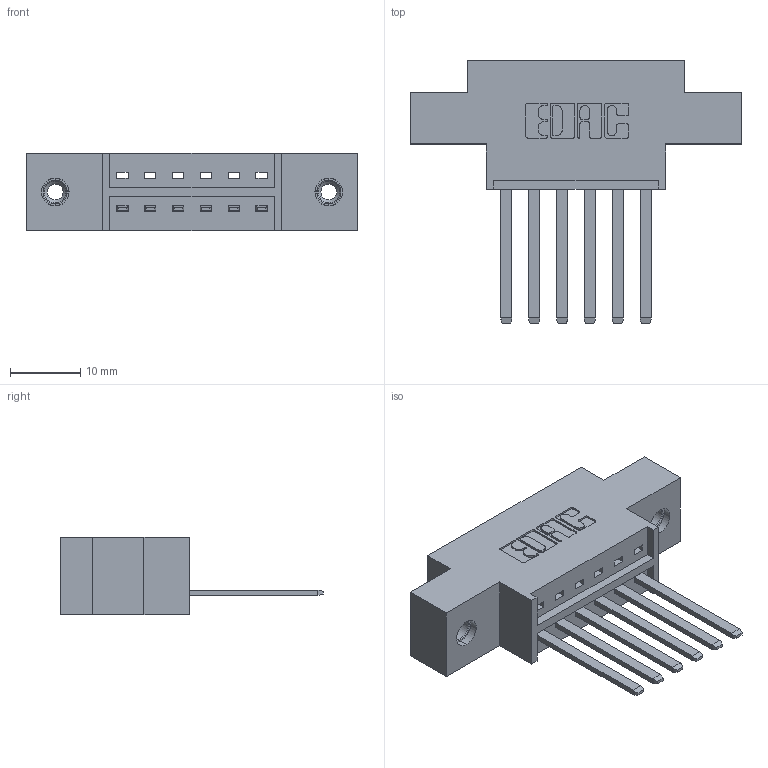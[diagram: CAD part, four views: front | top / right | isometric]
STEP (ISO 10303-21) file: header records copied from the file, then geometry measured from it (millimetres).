
FILE_DESCRIPTION (( 'STEP AP203' ), '1' );
FILE_NAME ('336-006-541-608.STEP', '2020-08-07T19:13:53', ( '' ), ( '' ), 'SwSTEP 2.0', 'SolidWorks 2020', '' );
FILE_SCHEMA (( 'CONFIG_CONTROL_DESIGN' ));
Length unit declared in the file: inch
Products named in the file (4): 345-250-001_345-250-003-102; 336-290-001_336-290-541; 336 Part_Offset - .156 Dia - TI; 336-006-541-608
Assembly tree (9 placements, depth 2):
  336-006-541-608
    336 Part_Offset - .156 Dia - TI
    336-290-001_336-290-541  x6
    345-250-001_345-250-003-102  x2
Bounding box: 47.17 x 37.34 x 11.1 mm (x, y, z)
Volume: 5825.1 mm3; surface area: 5990.3 mm2
Topology: 9 solids, 9 shells, 478 faces, 1383 edges, 910 vertices
Faces by surface type: plane 310, cylinder 152, cone 12, torus 4
Entity records: 10153 total; most frequent: CARTESIAN_POINT 1830, ORIENTED_EDGE 1666, DIRECTION 1551, EDGE_CURVE 833, LINE 681, VECTOR 681, VERTEX_POINT 550, AXIS2_PLACEMENT_3D 435
